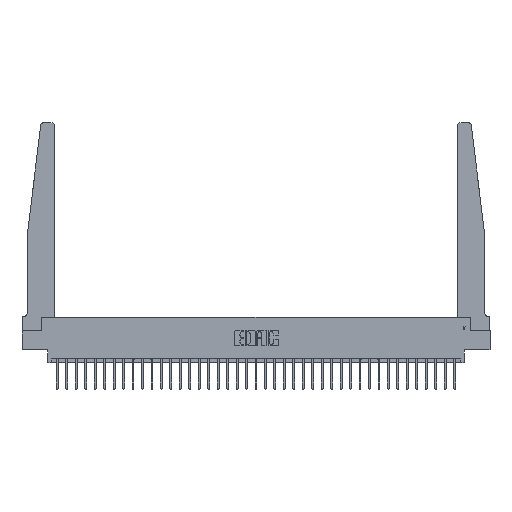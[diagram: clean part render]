
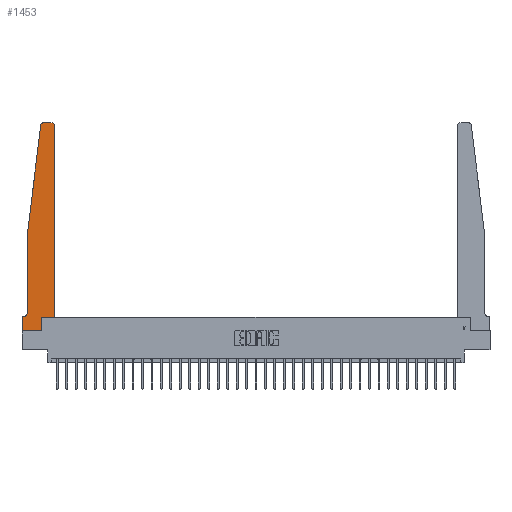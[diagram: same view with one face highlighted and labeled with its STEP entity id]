
A CAD part, top view. The second image highlights one B-rep face of the part: STEP entity #1453.
In plain terms, the highlighted planar face has unit normal (0, 0, 1).
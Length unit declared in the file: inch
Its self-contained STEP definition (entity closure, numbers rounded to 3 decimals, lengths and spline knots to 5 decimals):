
#314 = EDGE_CURVE ( 'NONE', #16873, #13008, #30745, .T. ) ;
#630 = VECTOR ( 'NONE', #16768, 39.37008 ) ;
#754 = DIRECTION ( 'NONE',  ( 0., 0., 1. ) ) ;
#1453 = ADVANCED_FACE ( 'NONE', ( #31948 ), #3776, .T. ) ;
#1890 = ORIENTED_EDGE ( 'NONE', *, *, #2305, .T. ) ;
#2305 = EDGE_CURVE ( 'NONE', #17629, #7092, #26912, .T. ) ;
#2854 = AXIS2_PLACEMENT_3D ( 'NONE', #20425, #30700, #17572 ) ;
#2881 = VECTOR ( 'NONE', #26267, 39.37008 ) ;
#3050 = LINE ( 'NONE', #7934, #9927 ) ;
#3253 = CIRCLE ( 'NONE', #28604, 0.03 ) ;
#3292 = CARTESIAN_POINT ( 'NONE',  ( 0., 0., 0.37 ) ) ;
#3776 = PLANE ( 'NONE',  #19523 ) ;
#4338 = CARTESIAN_POINT ( 'NONE',  ( 0.395, 2.75, 0.37 ) ) ;
#4554 = CARTESIAN_POINT ( 'NONE',  ( 0., 0., 0.37 ) ) ;
#4861 = VERTEX_POINT ( 'NONE', #6569 ) ;
#5212 = LINE ( 'NONE', #28500, #31672 ) ;
#5543 = CIRCLE ( 'NONE', #2854, 0.05 ) ;
#6017 = CARTESIAN_POINT ( 'NONE',  ( 0.24675, 2.72367, 0.37 ) ) ;
#6085 = ORIENTED_EDGE ( 'NONE', *, *, #15797, .T. ) ;
#6091 = EDGE_CURVE ( 'NONE', #21286, #16873, #23693, .T. ) ;
#6569 = CARTESIAN_POINT ( 'NONE',  ( 0.2605, 0.18, 0.37 ) ) ;
#7092 = VERTEX_POINT ( 'NONE', #4338 ) ;
#7096 = CARTESIAN_POINT ( 'NONE',  ( 0.27653, 2.75, 0.37 ) ) ;
#7874 = CARTESIAN_POINT ( 'NONE',  ( 0.065, 0.1875, 0.37 ) ) ;
#7934 = CARTESIAN_POINT ( 'NONE',  ( 0.2605, 0.18, 0.37 ) ) ;
#8045 = AXIS2_PLACEMENT_3D ( 'NONE', #12608, #20388, #27806 ) ;
#8217 = CARTESIAN_POINT ( 'NONE',  ( 0.425, 0.18, 0.37 ) ) ;
#8310 = DIRECTION ( 'NONE',  ( -0.122, -0.992, 0. ) ) ;
#8320 = CARTESIAN_POINT ( 'NONE',  ( 0.425, 0.18, 0.37 ) ) ;
#8506 = EDGE_CURVE ( 'NONE', #7092, #20550, #5212, .T. ) ;
#8555 = ORIENTED_EDGE ( 'NONE', *, *, #21298, .T. ) ;
#8665 = LINE ( 'NONE', #19149, #15825 ) ;
#8829 = DIRECTION ( 'NONE',  ( 1., 0., 0. ) ) ;
#9031 = DIRECTION ( 'NONE',  ( 1., 0., 0. ) ) ;
#9721 = ORIENTED_EDGE ( 'NONE', *, *, #24112, .T. ) ;
#9927 = VECTOR ( 'NONE', #13004, 39.37008 ) ;
#11524 = CARTESIAN_POINT ( 'NONE',  ( 0., 0.1875, 0.37 ) ) ;
#11764 = CARTESIAN_POINT ( 'NONE',  ( 0., 0.1875, 0.37 ) ) ;
#11857 = LINE ( 'NONE', #7874, #2881 ) ;
#12608 = CARTESIAN_POINT ( 'NONE',  ( 0.395, 2.72, 0.37 ) ) ;
#13004 = DIRECTION ( 'NONE',  ( 0., 1., 0. ) ) ;
#13008 = VERTEX_POINT ( 'NONE', #22260 ) ;
#13293 = CARTESIAN_POINT ( 'NONE',  ( 0.065, 1.25, 0.37 ) ) ;
#14284 = ORIENTED_EDGE ( 'NONE', *, *, #24590, .T. ) ;
#14635 = EDGE_LOOP ( 'NONE', ( #27686, #8555, #17232, #25160, #9721, #14284, #31442, #31917, #31151, #6085, #18749, #1890 ) ) ;
#15409 = LINE ( 'NONE', #15569, #32988 ) ;
#15569 = CARTESIAN_POINT ( 'NONE',  ( 0.425, 0.18, 0.37 ) ) ;
#15797 = EDGE_CURVE ( 'NONE', #4861, #25937, #15409, .T. ) ;
#15825 = VECTOR ( 'NONE', #29427, 39.37008 ) ;
#16407 = EDGE_CURVE ( 'NONE', #17590, #4861, #3050, .T. ) ;
#16768 = DIRECTION ( 'NONE',  ( 0., 1., 0. ) ) ;
#16873 = VERTEX_POINT ( 'NONE', #13293 ) ;
#17232 = ORIENTED_EDGE ( 'NONE', *, *, #6091, .T. ) ;
#17572 = DIRECTION ( 'NONE',  ( -1., 0., 0. ) ) ;
#17590 = VERTEX_POINT ( 'NONE', #28376 ) ;
#17629 = VERTEX_POINT ( 'NONE', #17764 ) ;
#17764 = CARTESIAN_POINT ( 'NONE',  ( 0.425, 2.72, 0.37 ) ) ;
#18033 = VECTOR ( 'NONE', #23894, 39.37008 ) ;
#18486 = LINE ( 'NONE', #8320, #630 ) ;
#18749 = ORIENTED_EDGE ( 'NONE', *, *, #18811, .T. ) ;
#18811 = EDGE_CURVE ( 'NONE', #25937, #17629, #18486, .T. ) ;
#18864 = CARTESIAN_POINT ( 'NONE',  ( 0.27653, 2.72, 0.37 ) ) ;
#19149 = CARTESIAN_POINT ( 'NONE',  ( 0., 0., 0.37 ) ) ;
#19523 = AXIS2_PLACEMENT_3D ( 'NONE', #11524, #754, #8829 ) ;
#19610 = VERTEX_POINT ( 'NONE', #11764 ) ;
#19725 = VECTOR ( 'NONE', #8310, 39.37008 ) ;
#20317 = DIRECTION ( 'NONE',  ( 1., 0., 0. ) ) ;
#20388 = DIRECTION ( 'NONE',  ( 0., 0., 1. ) ) ;
#20425 = CARTESIAN_POINT ( 'NONE',  ( 0.015, 0.2375, 0.37 ) ) ;
#20550 = VERTEX_POINT ( 'NONE', #7096 ) ;
#21286 = VERTEX_POINT ( 'NONE', #6017 ) ;
#21298 = EDGE_CURVE ( 'NONE', #20550, #21286, #3253, .T. ) ;
#22260 = CARTESIAN_POINT ( 'NONE',  ( 0.065, 0.2375, 0.37 ) ) ;
#22687 = VERTEX_POINT ( 'NONE', #4554 ) ;
#23029 = CARTESIAN_POINT ( 'NONE',  ( 0.065, 1.25, 0.37 ) ) ;
#23693 = LINE ( 'NONE', #23029, #19725 ) ;
#23894 = DIRECTION ( 'NONE',  ( 1., 0., 0. ) ) ;
#24112 = EDGE_CURVE ( 'NONE', #13008, #31653, #5543, .T. ) ;
#24590 = EDGE_CURVE ( 'NONE', #31653, #19610, #11857, .T. ) ;
#25081 = EDGE_CURVE ( 'NONE', #19610, #22687, #8665, .T. ) ;
#25160 = ORIENTED_EDGE ( 'NONE', *, *, #314, .T. ) ;
#25805 = DIRECTION ( 'NONE',  ( -1., 0., 0. ) ) ;
#25937 = VERTEX_POINT ( 'NONE', #8217 ) ;
#26267 = DIRECTION ( 'NONE',  ( -1., 0., 0. ) ) ;
#26410 = LINE ( 'NONE', #3292, #18033 ) ;
#26912 = CIRCLE ( 'NONE', #8045, 0.03 ) ;
#27686 = ORIENTED_EDGE ( 'NONE', *, *, #8506, .T. ) ;
#27806 = DIRECTION ( 'NONE',  ( 1., 0., 0. ) ) ;
#28111 = EDGE_CURVE ( 'NONE', #22687, #17590, #26410, .T. ) ;
#28376 = CARTESIAN_POINT ( 'NONE',  ( 0.2605, 0., 0.37 ) ) ;
#28500 = CARTESIAN_POINT ( 'NONE',  ( 0.25, 2.75, 0.37 ) ) ;
#28604 = AXIS2_PLACEMENT_3D ( 'NONE', #18864, #29796, #9031 ) ;
#28701 = VECTOR ( 'NONE', #30564, 39.37008 ) ;
#29005 = CARTESIAN_POINT ( 'NONE',  ( 0.065, 1.25, 0.37 ) ) ;
#29427 = DIRECTION ( 'NONE',  ( 0., -1., 0. ) ) ;
#29796 = DIRECTION ( 'NONE',  ( 0., 0., 1. ) ) ;
#30564 = DIRECTION ( 'NONE',  ( 0., -1., 0. ) ) ;
#30700 = DIRECTION ( 'NONE',  ( 0., 0., -1. ) ) ;
#30745 = LINE ( 'NONE', #29005, #28701 ) ;
#31151 = ORIENTED_EDGE ( 'NONE', *, *, #16407, .T. ) ;
#31442 = ORIENTED_EDGE ( 'NONE', *, *, #25081, .T. ) ;
#31653 = VERTEX_POINT ( 'NONE', #32089 ) ;
#31672 = VECTOR ( 'NONE', #25805, 39.37008 ) ;
#31917 = ORIENTED_EDGE ( 'NONE', *, *, #28111, .T. ) ;
#31948 = FACE_OUTER_BOUND ( 'NONE', #14635, .T. ) ;
#32089 = CARTESIAN_POINT ( 'NONE',  ( 0.015, 0.1875, 0.37 ) ) ;
#32988 = VECTOR ( 'NONE', #20317, 39.37008 ) ;
